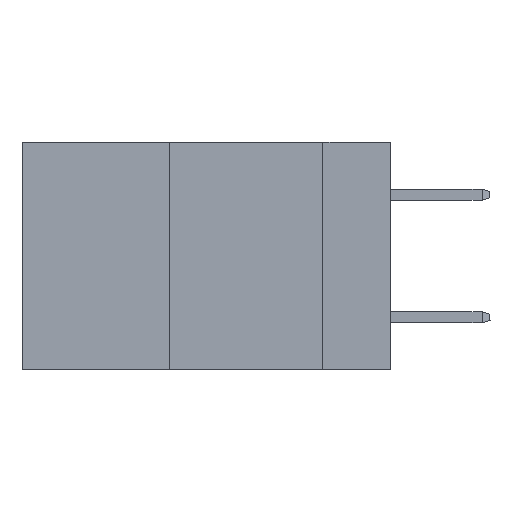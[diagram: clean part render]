
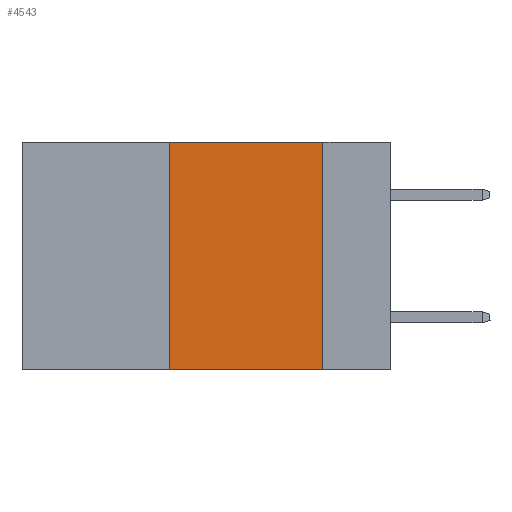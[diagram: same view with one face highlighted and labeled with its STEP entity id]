
A CAD part, left-side view. The second image highlights one B-rep face of the part: STEP entity #4543.
In plain terms, the highlighted planar face has unit normal (-1, 0, 0).
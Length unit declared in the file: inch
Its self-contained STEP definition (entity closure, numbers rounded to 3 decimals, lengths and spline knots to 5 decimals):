
#129 = DIRECTION ( 'NONE',  ( 0., 0., -1. ) ) ;
#471 = DIRECTION ( 'NONE',  ( 1., 0., 0. ) ) ;
#867 = VERTEX_POINT ( 'NONE', #12809 ) ;
#2894 = ORIENTED_EDGE ( 'NONE', *, *, #12608, .F. ) ;
#3498 = ORIENTED_EDGE ( 'NONE', *, *, #6183, .T. ) ;
#4492 = LINE ( 'NONE', #13112, #5985 ) ;
#4510 = ORIENTED_EDGE ( 'NONE', *, *, #12182, .F. ) ;
#4543 = ADVANCED_FACE ( 'NONE', ( #20126 ), #11833, .F. ) ;
#5941 = EDGE_CURVE ( 'NONE', #8562, #14004, #8152, .T. ) ;
#5985 = VECTOR ( 'NONE', #12935, 39.37008 ) ;
#6183 = EDGE_CURVE ( 'NONE', #8562, #20357, #4492, .T. ) ;
#6241 = DIRECTION ( 'NONE',  ( 0., 0., 1. ) ) ;
#7762 = DIRECTION ( 'NONE',  ( 0., 0., -1. ) ) ;
#8025 = VECTOR ( 'NONE', #16654, 39.37008 ) ;
#8152 = LINE ( 'NONE', #17924, #23151 ) ;
#8562 = VERTEX_POINT ( 'NONE', #16647 ) ;
#8890 = CARTESIAN_POINT ( 'NONE',  ( 0., 0.6, 0. ) ) ;
#9569 = VECTOR ( 'NONE', #7762, 39.37008 ) ;
#11833 = PLANE ( 'NONE',  #22399 ) ;
#12182 = EDGE_CURVE ( 'NONE', #867, #20357, #17820, .T. ) ;
#12597 = EDGE_LOOP ( 'NONE', ( #4510, #2894, #14881, #3498 ) ) ;
#12608 = EDGE_CURVE ( 'NONE', #14004, #867, #23620, .T. ) ;
#12809 = CARTESIAN_POINT ( 'NONE',  ( 0., 0.11, 0. ) ) ;
#12935 = DIRECTION ( 'NONE',  ( 0., -1., 0. ) ) ;
#13112 = CARTESIAN_POINT ( 'NONE',  ( 0., 0.6, -0.37 ) ) ;
#14004 = VERTEX_POINT ( 'NONE', #14170 ) ;
#14170 = CARTESIAN_POINT ( 'NONE',  ( 0., 0.36, 0. ) ) ;
#14881 = ORIENTED_EDGE ( 'NONE', *, *, #5941, .F. ) ;
#16647 = CARTESIAN_POINT ( 'NONE',  ( 0., 0.36, -0.37 ) ) ;
#16654 = DIRECTION ( 'NONE',  ( 0., -1., 0. ) ) ;
#17767 = CARTESIAN_POINT ( 'NONE',  ( 0., 0.11, 0. ) ) ;
#17820 = LINE ( 'NONE', #17767, #9569 ) ;
#17924 = CARTESIAN_POINT ( 'NONE',  ( 0., 0.36, 0. ) ) ;
#20126 = FACE_OUTER_BOUND ( 'NONE', #12597, .T. ) ;
#20357 = VERTEX_POINT ( 'NONE', #24641 ) ;
#22399 = AXIS2_PLACEMENT_3D ( 'NONE', #23911, #471, #129 ) ;
#23151 = VECTOR ( 'NONE', #6241, 39.37008 ) ;
#23620 = LINE ( 'NONE', #8890, #8025 ) ;
#23911 = CARTESIAN_POINT ( 'NONE',  ( 0., 0.6, 0. ) ) ;
#24641 = CARTESIAN_POINT ( 'NONE',  ( 0., 0.11, -0.37 ) ) ;
